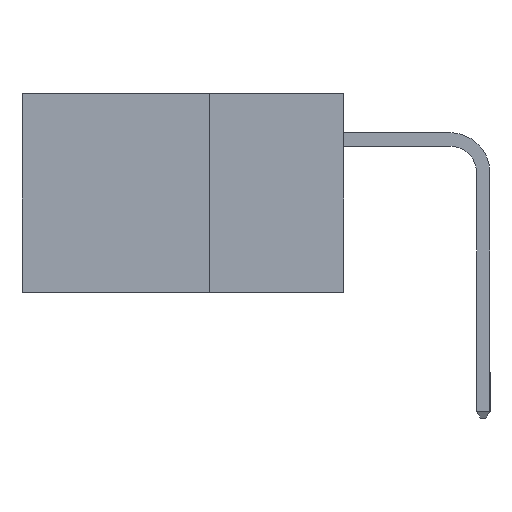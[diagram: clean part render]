
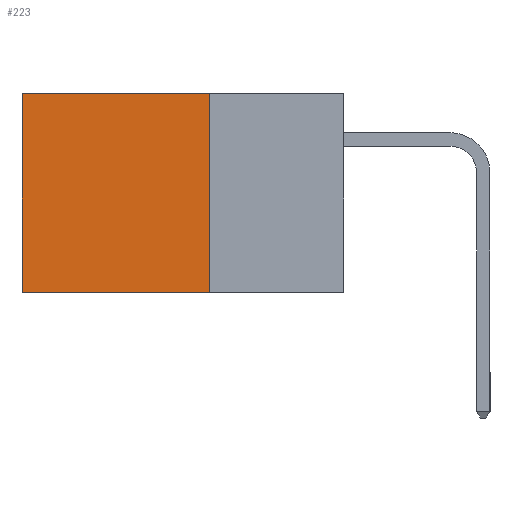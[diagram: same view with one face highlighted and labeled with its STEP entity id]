
A CAD part, left-side view. The second image highlights one B-rep face of the part: STEP entity #223.
In plain terms, the highlighted planar face has unit normal (-1, 0, 0).
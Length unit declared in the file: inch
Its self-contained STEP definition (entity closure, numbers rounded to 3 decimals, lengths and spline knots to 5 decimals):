
#107 = EDGE_CURVE ( 'NONE', #929, #6557, #3953, .T. ) ;
#143 = CARTESIAN_POINT ( 'NONE',  ( 0.298, 0.25, 0. ) ) ;
#223 = ADVANCED_FACE ( 'NONE', ( #257 ), #4256, .F. ) ;
#257 = FACE_OUTER_BOUND ( 'NONE', #6100, .T. ) ;
#384 = CARTESIAN_POINT ( 'NONE',  ( 0.298, 0.6, -0.37 ) ) ;
#488 = DIRECTION ( 'NONE',  ( 1., 0., 0. ) ) ;
#627 = ORIENTED_EDGE ( 'NONE', *, *, #7615, .F. ) ;
#929 = VERTEX_POINT ( 'NONE', #8296 ) ;
#1145 = CARTESIAN_POINT ( 'NONE',  ( 0.298, 0.25, -0.37 ) ) ;
#1439 = VECTOR ( 'NONE', #7818, 39.37008 ) ;
#1971 = AXIS2_PLACEMENT_3D ( 'NONE', #10833, #488, #7163 ) ;
#2145 = VECTOR ( 'NONE', #5911, 39.37008 ) ;
#2308 = VECTOR ( 'NONE', #6745, 39.37008 ) ;
#2981 = VECTOR ( 'NONE', #11499, 39.37008 ) ;
#3475 = VERTEX_POINT ( 'NONE', #7613 ) ;
#3812 = CARTESIAN_POINT ( 'NONE',  ( 0.298, 0.25, 0. ) ) ;
#3953 = LINE ( 'NONE', #10701, #1439 ) ;
#4256 = PLANE ( 'NONE',  #1971 ) ;
#4289 = ORIENTED_EDGE ( 'NONE', *, *, #7440, .F. ) ;
#4515 = EDGE_CURVE ( 'NONE', #8193, #929, #5501, .T. ) ;
#5501 = LINE ( 'NONE', #143, #2981 ) ;
#5911 = DIRECTION ( 'NONE',  ( 0., 0., -1. ) ) ;
#6100 = EDGE_LOOP ( 'NONE', ( #8756, #4289, #627, #9575 ) ) ;
#6557 = VERTEX_POINT ( 'NONE', #384 ) ;
#6745 = DIRECTION ( 'NONE',  ( 0., 1., 0. ) ) ;
#7163 = DIRECTION ( 'NONE',  ( 0., 0., -1. ) ) ;
#7360 = LINE ( 'NONE', #1145, #2308 ) ;
#7440 = EDGE_CURVE ( 'NONE', #3475, #6557, #7360, .T. ) ;
#7613 = CARTESIAN_POINT ( 'NONE',  ( 0.298, 0.25, -0.37 ) ) ;
#7615 = EDGE_CURVE ( 'NONE', #8193, #3475, #11603, .T. ) ;
#7818 = DIRECTION ( 'NONE',  ( 0., 0., -1. ) ) ;
#8193 = VERTEX_POINT ( 'NONE', #3812 ) ;
#8296 = CARTESIAN_POINT ( 'NONE',  ( 0.298, 0.6, 0. ) ) ;
#8756 = ORIENTED_EDGE ( 'NONE', *, *, #107, .T. ) ;
#9575 = ORIENTED_EDGE ( 'NONE', *, *, #4515, .T. ) ;
#9837 = CARTESIAN_POINT ( 'NONE',  ( 0.298, 0.25, 0. ) ) ;
#10701 = CARTESIAN_POINT ( 'NONE',  ( 0.298, 0.6, 0. ) ) ;
#10833 = CARTESIAN_POINT ( 'NONE',  ( 0.298, 0.25, 0. ) ) ;
#11499 = DIRECTION ( 'NONE',  ( 0., 1., 0. ) ) ;
#11603 = LINE ( 'NONE', #9837, #2145 ) ;
